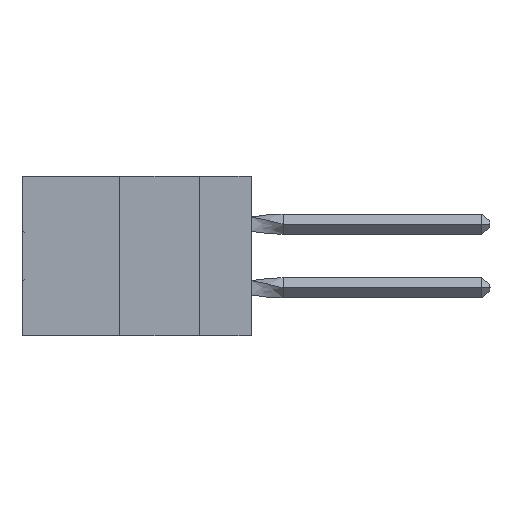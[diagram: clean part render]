
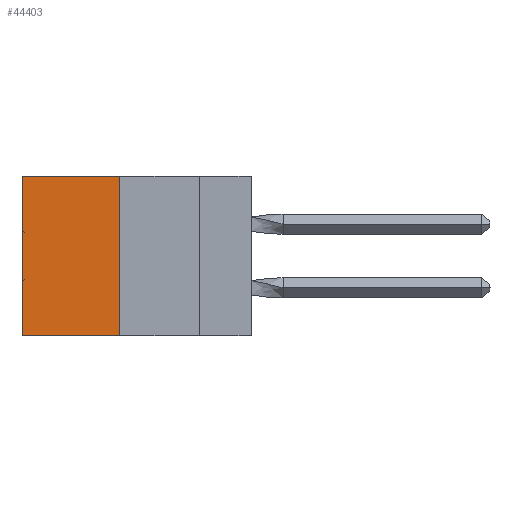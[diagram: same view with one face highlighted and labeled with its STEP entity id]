
A CAD part, left-side view. The second image highlights one B-rep face of the part: STEP entity #44403.
In plain terms, the highlighted planar face has unit normal (-1, 0, 0).
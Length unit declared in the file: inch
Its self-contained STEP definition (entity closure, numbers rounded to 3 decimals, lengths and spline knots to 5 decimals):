
#417 = LINE ( 'NONE', #45980, #22771 ) ;
#7328 = CARTESIAN_POINT ( 'NONE',  ( 0.305, 0.413, -0.5 ) ) ;
#9233 = LINE ( 'NONE', #25917, #50219 ) ;
#10709 = ORIENTED_EDGE ( 'NONE', *, *, #38871, .T. ) ;
#11333 = DIRECTION ( 'NONE',  ( 0., 0., -1. ) ) ;
#13191 = EDGE_CURVE ( 'NONE', #15670, #26594, #417, .T. ) ;
#15323 = DIRECTION ( 'NONE',  ( 1., 0., 0. ) ) ;
#15670 = VERTEX_POINT ( 'NONE', #48243 ) ;
#17193 = AXIS2_PLACEMENT_3D ( 'NONE', #7328, #15323, #11333 ) ;
#17227 = LINE ( 'NONE', #30771, #37143 ) ;
#22771 = VECTOR ( 'NONE', #25641, 39.37008 ) ;
#25641 = DIRECTION ( 'NONE',  ( 0., 1., 0. ) ) ;
#25917 = CARTESIAN_POINT ( 'NONE',  ( 0.305, 0.413, -0.5 ) ) ;
#26011 = EDGE_LOOP ( 'NONE', ( #10709, #41398, #48401, #26456 ) ) ;
#26456 = ORIENTED_EDGE ( 'NONE', *, *, #13191, .T. ) ;
#26594 = VERTEX_POINT ( 'NONE', #44271 ) ;
#26672 = DIRECTION ( 'NONE',  ( 0., 1., 0. ) ) ;
#27014 = CARTESIAN_POINT ( 'NONE',  ( 0.305, 0.413, -0.5 ) ) ;
#28090 = FACE_OUTER_BOUND ( 'NONE', #26011, .T. ) ;
#28333 = VERTEX_POINT ( 'NONE', #45355 ) ;
#30771 = CARTESIAN_POINT ( 'NONE',  ( 0.305, 0.72, -0.5 ) ) ;
#34540 = LINE ( 'NONE', #27014, #38302 ) ;
#37143 = VECTOR ( 'NONE', #41927, 39.37008 ) ;
#38302 = VECTOR ( 'NONE', #26672, 39.37008 ) ;
#38871 = EDGE_CURVE ( 'NONE', #26594, #28333, #17227, .T. ) ;
#41114 = EDGE_CURVE ( 'NONE', #15670, #44258, #9233, .T. ) ;
#41398 = ORIENTED_EDGE ( 'NONE', *, *, #48063, .F. ) ;
#41927 = DIRECTION ( 'NONE',  ( 0., 0., -1. ) ) ;
#43137 = PLANE ( 'NONE',  #17193 ) ;
#44258 = VERTEX_POINT ( 'NONE', #46288 ) ;
#44271 = CARTESIAN_POINT ( 'NONE',  ( 0.305, 0.72, 0. ) ) ;
#44403 = ADVANCED_FACE ( 'NONE', ( #28090 ), #43137, .F. ) ;
#45355 = CARTESIAN_POINT ( 'NONE',  ( 0.305, 0.72, -0.5 ) ) ;
#45980 = CARTESIAN_POINT ( 'NONE',  ( 0.305, 0.413, 0. ) ) ;
#46288 = CARTESIAN_POINT ( 'NONE',  ( 0.305, 0.413, -0.5 ) ) ;
#46422 = DIRECTION ( 'NONE',  ( 0., 0., -1. ) ) ;
#48063 = EDGE_CURVE ( 'NONE', #44258, #28333, #34540, .T. ) ;
#48243 = CARTESIAN_POINT ( 'NONE',  ( 0.305, 0.413, 0. ) ) ;
#48401 = ORIENTED_EDGE ( 'NONE', *, *, #41114, .F. ) ;
#50219 = VECTOR ( 'NONE', #46422, 39.37008 ) ;
